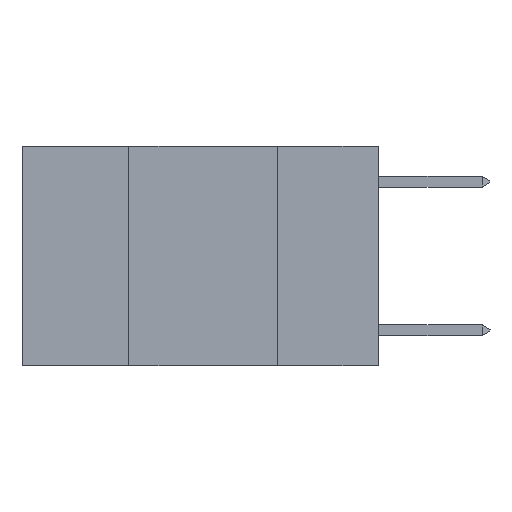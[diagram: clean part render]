
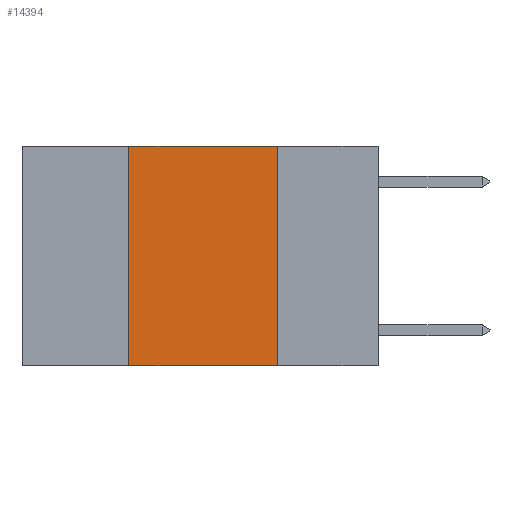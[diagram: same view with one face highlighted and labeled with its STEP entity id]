
A CAD part, left-side view. The second image highlights one B-rep face of the part: STEP entity #14394.
In plain terms, the highlighted planar face has unit normal (-1, 0, 0).
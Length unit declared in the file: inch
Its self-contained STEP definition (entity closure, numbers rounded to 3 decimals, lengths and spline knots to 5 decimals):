
#555 = VECTOR ( 'NONE', #3900, 39.37008 ) ;
#1227 = CARTESIAN_POINT ( 'NONE',  ( 0., 0.6, -0.37 ) ) ;
#1267 = DIRECTION ( 'NONE',  ( 0., -1., 0. ) ) ;
#1698 = LINE ( 'NONE', #1227, #5733 ) ;
#3311 = DIRECTION ( 'NONE',  ( 0., 0., -1. ) ) ;
#3900 = DIRECTION ( 'NONE',  ( 0., -1., 0. ) ) ;
#3977 = CARTESIAN_POINT ( 'NONE',  ( 0., 0.6, 0. ) ) ;
#4873 = ORIENTED_EDGE ( 'NONE', *, *, #10608, .T. ) ;
#5533 = VECTOR ( 'NONE', #18617, 39.37008 ) ;
#5733 = VECTOR ( 'NONE', #1267, 39.37008 ) ;
#6417 = EDGE_CURVE ( 'NONE', #12825, #14123, #8508, .T. ) ;
#6606 = CARTESIAN_POINT ( 'NONE',  ( 0., 0.42, 0. ) ) ;
#6628 = DIRECTION ( 'NONE',  ( 0., 0., 1. ) ) ;
#6839 = VERTEX_POINT ( 'NONE', #17058 ) ;
#7798 = EDGE_LOOP ( 'NONE', ( #16687, #17624, #8924, #4873 ) ) ;
#8508 = LINE ( 'NONE', #6606, #15550 ) ;
#8924 = ORIENTED_EDGE ( 'NONE', *, *, #6417, .F. ) ;
#9904 = AXIS2_PLACEMENT_3D ( 'NONE', #15345, #12451, #3311 ) ;
#10427 = EDGE_CURVE ( 'NONE', #14123, #11061, #16590, .T. ) ;
#10608 = EDGE_CURVE ( 'NONE', #12825, #6839, #1698, .T. ) ;
#10919 = PLANE ( 'NONE',  #9904 ) ;
#11061 = VERTEX_POINT ( 'NONE', #15846 ) ;
#12451 = DIRECTION ( 'NONE',  ( 1., 0., 0. ) ) ;
#12740 = CARTESIAN_POINT ( 'NONE',  ( 0., 0.17, 0. ) ) ;
#12825 = VERTEX_POINT ( 'NONE', #15321 ) ;
#14123 = VERTEX_POINT ( 'NONE', #17681 ) ;
#14394 = ADVANCED_FACE ( 'NONE', ( #16035 ), #10919, .F. ) ;
#15321 = CARTESIAN_POINT ( 'NONE',  ( 0., 0.42, -0.37 ) ) ;
#15345 = CARTESIAN_POINT ( 'NONE',  ( 0., 0.6, 0. ) ) ;
#15550 = VECTOR ( 'NONE', #6628, 39.37008 ) ;
#15846 = CARTESIAN_POINT ( 'NONE',  ( 0., 0.17, 0. ) ) ;
#16035 = FACE_OUTER_BOUND ( 'NONE', #7798, .T. ) ;
#16590 = LINE ( 'NONE', #3977, #555 ) ;
#16687 = ORIENTED_EDGE ( 'NONE', *, *, #17338, .F. ) ;
#17058 = CARTESIAN_POINT ( 'NONE',  ( 0., 0.17, -0.37 ) ) ;
#17338 = EDGE_CURVE ( 'NONE', #11061, #6839, #17518, .T. ) ;
#17518 = LINE ( 'NONE', #12740, #5533 ) ;
#17624 = ORIENTED_EDGE ( 'NONE', *, *, #10427, .F. ) ;
#17681 = CARTESIAN_POINT ( 'NONE',  ( 0., 0.42, 0. ) ) ;
#18617 = DIRECTION ( 'NONE',  ( 0., 0., -1. ) ) ;
